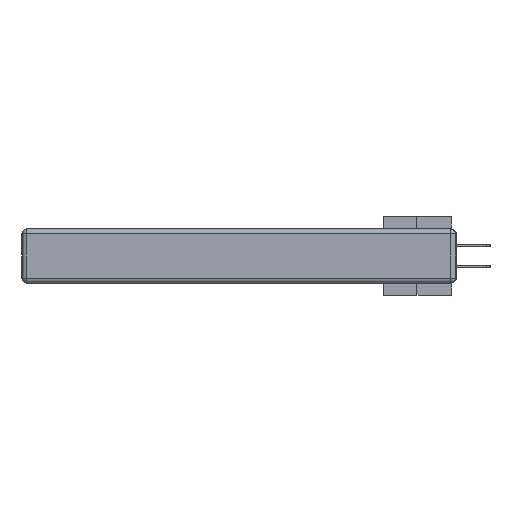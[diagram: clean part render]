
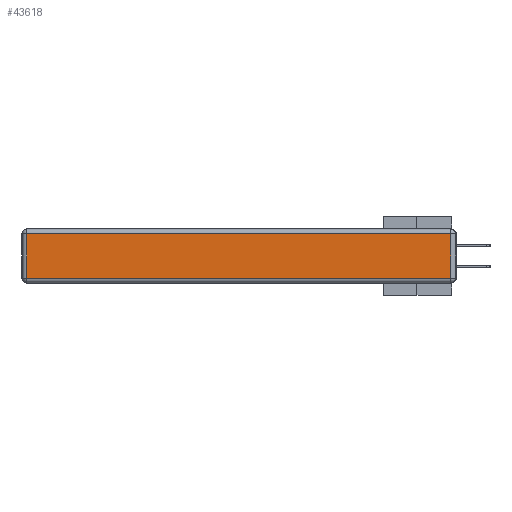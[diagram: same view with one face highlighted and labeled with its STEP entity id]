
A CAD part, left-side view. The second image highlights one B-rep face of the part: STEP entity #43618.
In plain terms, the highlighted planar face has unit normal (-1, 0, 0).
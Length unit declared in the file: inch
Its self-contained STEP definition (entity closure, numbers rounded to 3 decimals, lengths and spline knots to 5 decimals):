
#332 = CARTESIAN_POINT ( 'NONE',  ( 0., 2.72, -0.343 ) ) ;
#857 = CARTESIAN_POINT ( 'NONE',  ( 0., 2.72, -0.313 ) ) ;
#1330 = VECTOR ( 'NONE', #32289, 39.37008 ) ;
#1649 = VECTOR ( 'NONE', #26960, 39.37008 ) ;
#2494 = CARTESIAN_POINT ( 'NONE',  ( 0., 0.03, -0.343 ) ) ;
#3223 = VERTEX_POINT ( 'NONE', #30413 ) ;
#3483 = ORIENTED_EDGE ( 'NONE', *, *, #15079, .T. ) ;
#3661 = VECTOR ( 'NONE', #36081, 39.37008 ) ;
#5615 = EDGE_CURVE ( 'NONE', #23554, #20476, #26425, .T. ) ;
#6106 = CARTESIAN_POINT ( 'NONE',  ( 0., 2.75, -0.03 ) ) ;
#6239 = ORIENTED_EDGE ( 'NONE', *, *, #20381, .T. ) ;
#7146 = DIRECTION ( 'NONE',  ( 0., 1., 0. ) ) ;
#10837 = PLANE ( 'NONE',  #21455 ) ;
#10979 = DIRECTION ( 'NONE',  ( 0., 0., 1. ) ) ;
#11771 = ORIENTED_EDGE ( 'NONE', *, *, #5615, .T. ) ;
#12959 = CARTESIAN_POINT ( 'NONE',  ( 0., 0.03, -0.03 ) ) ;
#14239 = DIRECTION ( 'NONE',  ( -1., 0., 0. ) ) ;
#15079 = EDGE_CURVE ( 'NONE', #20759, #23554, #35094, .T. ) ;
#17913 = EDGE_LOOP ( 'NONE', ( #6239, #35414, #3483, #11771 ) ) ;
#19473 = LINE ( 'NONE', #2494, #1649 ) ;
#20381 = EDGE_CURVE ( 'NONE', #20476, #3223, #31538, .T. ) ;
#20476 = VERTEX_POINT ( 'NONE', #857 ) ;
#20759 = VERTEX_POINT ( 'NONE', #12959 ) ;
#21455 = AXIS2_PLACEMENT_3D ( 'NONE', #35755, #14239, #10979 ) ;
#23416 = FACE_OUTER_BOUND ( 'NONE', #17913, .T. ) ;
#23554 = VERTEX_POINT ( 'NONE', #34920 ) ;
#25591 = VECTOR ( 'NONE', #7146, 39.37008 ) ;
#26425 = LINE ( 'NONE', #332, #1330 ) ;
#26960 = DIRECTION ( 'NONE',  ( 0., 0., 1. ) ) ;
#30413 = CARTESIAN_POINT ( 'NONE',  ( 0., 0.03, -0.313 ) ) ;
#31538 = LINE ( 'NONE', #41479, #3661 ) ;
#32289 = DIRECTION ( 'NONE',  ( 0., 0., -1. ) ) ;
#34920 = CARTESIAN_POINT ( 'NONE',  ( 0., 2.72, -0.03 ) ) ;
#35094 = LINE ( 'NONE', #6106, #25591 ) ;
#35414 = ORIENTED_EDGE ( 'NONE', *, *, #42783, .T. ) ;
#35755 = CARTESIAN_POINT ( 'NONE',  ( 0., 0., -0.343 ) ) ;
#36081 = DIRECTION ( 'NONE',  ( 0., -1., 0. ) ) ;
#41479 = CARTESIAN_POINT ( 'NONE',  ( 0., 0., -0.313 ) ) ;
#42783 = EDGE_CURVE ( 'NONE', #3223, #20759, #19473, .T. ) ;
#43618 = ADVANCED_FACE ( 'NONE', ( #23416 ), #10837, .T. ) ;
